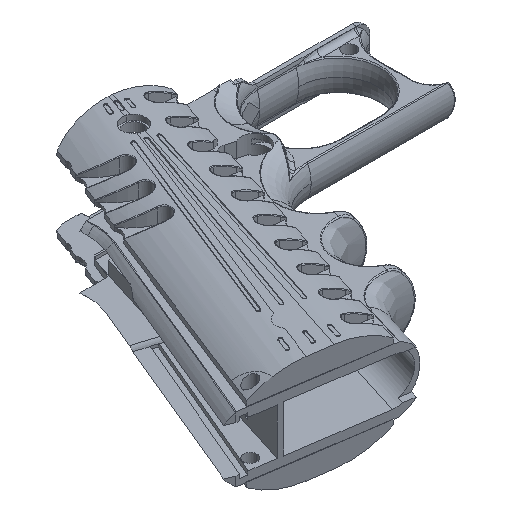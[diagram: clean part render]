
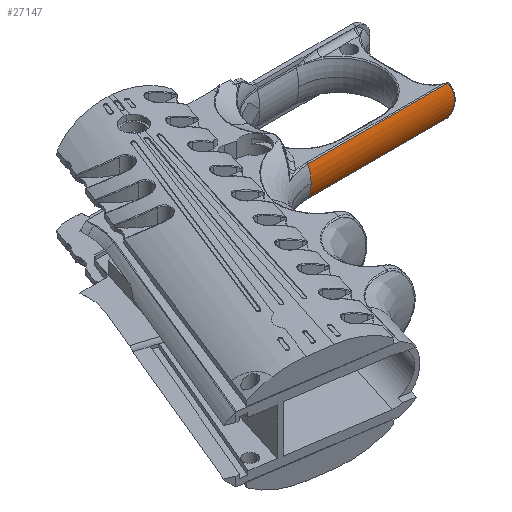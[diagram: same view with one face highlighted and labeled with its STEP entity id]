
A CAD part, isometric view. The second image highlights one B-rep face of the part: STEP entity #27147.
In plain terms, the highlighted cylindrical face has radius 10.414 mm (diameter 20.828 mm), a partial arc.
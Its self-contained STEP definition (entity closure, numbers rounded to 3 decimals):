
#1321 = CARTESIAN_POINT ( 'NONE',  ( 19.673, -35.853, 3.767 ) ) ;
#1411 = DIRECTION ( 'NONE',  ( 0., 0., -1. ) ) ;
#2355 = EDGE_CURVE ( 'NONE', #30997, #9044, #8135, .T. ) ;
#2428 = VECTOR ( 'NONE', #30406, 1000. ) ;
#2725 = EDGE_CURVE ( 'NONE', #18209, #32251, #24077, .T. ) ;
#3815 = EDGE_CURVE ( 'NONE', #25837, #9044, #13118, .T. ) ;
#4036 = CARTESIAN_POINT ( 'NONE',  ( 19.386, -35.556, -4.442 ) ) ;
#4146 = CARTESIAN_POINT ( 'NONE',  ( 19.386, -35.556, 4.442 ) ) ;
#4207 = AXIS2_PLACEMENT_3D ( 'NONE', #11598, #31357, #14428 ) ;
#4665 = EDGE_CURVE ( 'NONE', #32251, #30997, #5314, .T. ) ;
#4698 = CARTESIAN_POINT ( 'NONE',  ( 0.762, -35.556, -4.442 ) ) ;
#5292 = ORIENTED_EDGE ( 'NONE', *, *, #4665, .T. ) ;
#5314 = B_SPLINE_CURVE_WITH_KNOTS ( 'NONE', 3,
 ( #4036, #20909, #18069, #23738, #6821, #26607, #9684, #29449, #12535, #32320, #15382, #35156, #18184, #1321, #21037, #4146 ),
 .UNSPECIFIED., .F., .F.,
 ( 4, 2, 2, 2, 2, 2, 2, 4 ),
 ( 0., 0.002, 0.004, 0.005, 0.006, 0.007, 0.008, 0.009 ),
 .UNSPECIFIED. ) ;
#6821 = CARTESIAN_POINT ( 'NONE',  ( 20.242, -36.44, -1.56 ) ) ;
#7601 = ORIENTED_EDGE ( 'NONE', *, *, #23438, .F. ) ;
#8135 = LINE ( 'NONE', #10655, #2428 ) ;
#8616 = EDGE_LOOP ( 'NONE', ( #17700, #5292, #29289, #27597, #7601 ) ) ;
#8813 = DIRECTION ( 'NONE',  ( 0., 0., 1. ) ) ;
#9044 = VERTEX_POINT ( 'NONE', #20515 ) ;
#9639 = CYLINDRICAL_SURFACE ( 'NONE', #25782, 10.414 ) ;
#9684 = CARTESIAN_POINT ( 'NONE',  ( 20.348, -36.55, -0.397 ) ) ;
#10655 = CARTESIAN_POINT ( 'NONE',  ( 0.762, -35.556, 4.442 ) ) ;
#11598 = CARTESIAN_POINT ( 'NONE',  ( -22.268, -26.137, 0. ) ) ;
#12535 = CARTESIAN_POINT ( 'NONE',  ( 20.326, -36.528, 0.786 ) ) ;
#13118 = CIRCLE ( 'NONE', #4207, 10.414 ) ;
#14428 = DIRECTION ( 'NONE',  ( 0., 0., -1. ) ) ;
#14481 = CARTESIAN_POINT ( 'NONE',  ( -22.268, -36.551, 0. ) ) ;
#14648 = DIRECTION ( 'NONE',  ( -1., 0., 0. ) ) ;
#15382 = CARTESIAN_POINT ( 'NONE',  ( 20.178, -36.375, 1.942 ) ) ;
#15717 = VECTOR ( 'NONE', #24422, 1000. ) ;
#16087 = CARTESIAN_POINT ( 'NONE',  ( 19.386, -35.556, -4.442 ) ) ;
#17143 = FACE_OUTER_BOUND ( 'NONE', #8616, .T. ) ;
#17700 = ORIENTED_EDGE ( 'NONE', *, *, #2725, .T. ) ;
#17885 = CIRCLE ( 'NONE', #32783, 10.414 ) ;
#18069 = CARTESIAN_POINT ( 'NONE',  ( 19.928, -36.116, -3.076 ) ) ;
#18184 = CARTESIAN_POINT ( 'NONE',  ( 19.913, -36.1, 3.054 ) ) ;
#18209 = VERTEX_POINT ( 'NONE', #33615 ) ;
#18282 = DIRECTION ( 'NONE',  ( -1., 0., 0. ) ) ;
#20515 = CARTESIAN_POINT ( 'NONE',  ( -22.268, -35.556, 4.442 ) ) ;
#20909 = CARTESIAN_POINT ( 'NONE',  ( 19.688, -35.868, -3.78 ) ) ;
#21037 = CARTESIAN_POINT ( 'NONE',  ( 19.537, -35.712, 4.111 ) ) ;
#23438 = EDGE_CURVE ( 'NONE', #18209, #25837, #17885, .T. ) ;
#23738 = CARTESIAN_POINT ( 'NONE',  ( 20.178, -36.374, -1.947 ) ) ;
#24077 = LINE ( 'NONE', #4698, #15717 ) ;
#24422 = DIRECTION ( 'NONE',  ( 1., 0., 0. ) ) ;
#25782 = AXIS2_PLACEMENT_3D ( 'NONE', #31555, #14648, #8813 ) ;
#25837 = VERTEX_POINT ( 'NONE', #14481 ) ;
#26607 = CARTESIAN_POINT ( 'NONE',  ( 20.326, -36.528, -0.787 ) ) ;
#27147 = ADVANCED_FACE ( 'NONE', ( #17143 ), #9639, .T. ) ;
#27597 = ORIENTED_EDGE ( 'NONE', *, *, #3815, .F. ) ;
#29289 = ORIENTED_EDGE ( 'NONE', *, *, #2355, .T. ) ;
#29449 = CARTESIAN_POINT ( 'NONE',  ( 20.348, -36.551, 0.388 ) ) ;
#30406 = DIRECTION ( 'NONE',  ( -1., 0., 0. ) ) ;
#30997 = VERTEX_POINT ( 'NONE', #34394 ) ;
#31357 = DIRECTION ( 'NONE',  ( -1., 0., 0. ) ) ;
#31555 = CARTESIAN_POINT ( 'NONE',  ( 0.762, -26.137, 0. ) ) ;
#32251 = VERTEX_POINT ( 'NONE', #16087 ) ;
#32320 = CARTESIAN_POINT ( 'NONE',  ( 20.241, -36.44, 1.562 ) ) ;
#32783 = AXIS2_PLACEMENT_3D ( 'NONE', #35259, #18282, #1411 ) ;
#33615 = CARTESIAN_POINT ( 'NONE',  ( -22.268, -35.556, -4.442 ) ) ;
#34394 = CARTESIAN_POINT ( 'NONE',  ( 19.386, -35.556, 4.442 ) ) ;
#35156 = CARTESIAN_POINT ( 'NONE',  ( 20.014, -36.205, 2.688 ) ) ;
#35259 = CARTESIAN_POINT ( 'NONE',  ( -22.268, -26.137, 0. ) ) ;
